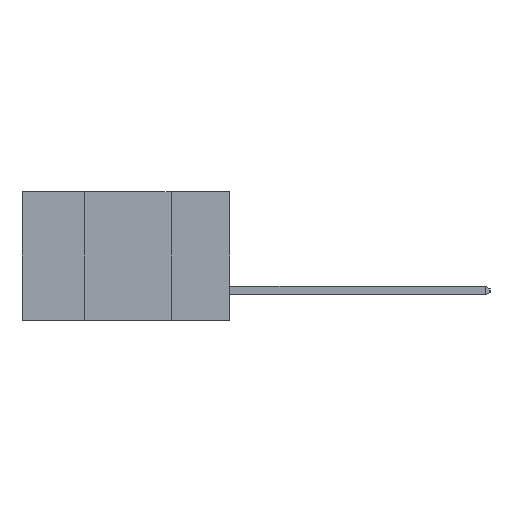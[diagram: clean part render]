
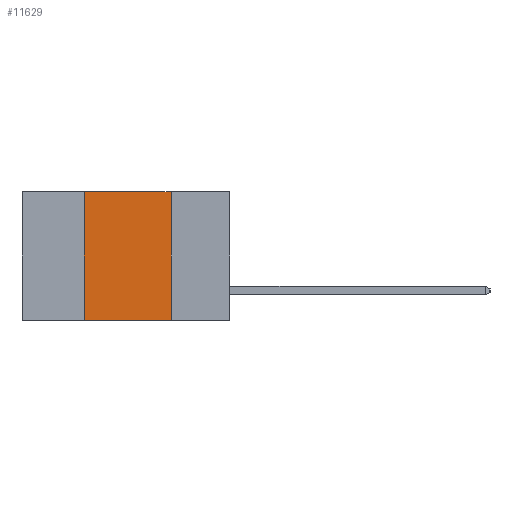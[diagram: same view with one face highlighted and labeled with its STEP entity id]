
A CAD part, left-side view. The second image highlights one B-rep face of the part: STEP entity #11629.
In plain terms, the highlighted planar face has unit normal (-1, 0, 0).
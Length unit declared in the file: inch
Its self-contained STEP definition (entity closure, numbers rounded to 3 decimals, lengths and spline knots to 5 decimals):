
#377 = CARTESIAN_POINT ( 'NONE',  ( 0., 0.42, 0. ) ) ;
#571 = DIRECTION ( 'NONE',  ( 0., -1., 0. ) ) ;
#684 = CARTESIAN_POINT ( 'NONE',  ( 0., 0.42, -0.37 ) ) ;
#943 = EDGE_LOOP ( 'NONE', ( #2612, #11514, #7344, #5136 ) ) ;
#1058 = CARTESIAN_POINT ( 'NONE',  ( 0., 0.6, -0.37 ) ) ;
#1068 = AXIS2_PLACEMENT_3D ( 'NONE', #4543, #5641, #13134 ) ;
#2128 = LINE ( 'NONE', #7784, #7578 ) ;
#2478 = EDGE_CURVE ( 'NONE', #11890, #4574, #3225, .T. ) ;
#2612 = ORIENTED_EDGE ( 'NONE', *, *, #4642, .F. ) ;
#3178 = EDGE_CURVE ( 'NONE', #11890, #9450, #10637, .T. ) ;
#3225 = LINE ( 'NONE', #1058, #5809 ) ;
#3262 = CARTESIAN_POINT ( 'NONE',  ( 0., 0.17, 0. ) ) ;
#3525 = DIRECTION ( 'NONE',  ( 0., 0., -1. ) ) ;
#4326 = CARTESIAN_POINT ( 'NONE',  ( 0., 0.42, 0. ) ) ;
#4514 = LINE ( 'NONE', #7840, #12747 ) ;
#4543 = CARTESIAN_POINT ( 'NONE',  ( 0., 0.6, 0. ) ) ;
#4574 = VERTEX_POINT ( 'NONE', #13069 ) ;
#4642 = EDGE_CURVE ( 'NONE', #6007, #4574, #4514, .T. ) ;
#4832 = DIRECTION ( 'NONE',  ( 0., 0., 1. ) ) ;
#5136 = ORIENTED_EDGE ( 'NONE', *, *, #2478, .T. ) ;
#5641 = DIRECTION ( 'NONE',  ( 1., 0., 0. ) ) ;
#5809 = VECTOR ( 'NONE', #571, 39.37008 ) ;
#6007 = VERTEX_POINT ( 'NONE', #3262 ) ;
#7032 = EDGE_CURVE ( 'NONE', #9450, #6007, #2128, .T. ) ;
#7344 = ORIENTED_EDGE ( 'NONE', *, *, #3178, .F. ) ;
#7578 = VECTOR ( 'NONE', #9942, 39.37008 ) ;
#7784 = CARTESIAN_POINT ( 'NONE',  ( 0., 0.6, 0. ) ) ;
#7840 = CARTESIAN_POINT ( 'NONE',  ( 0., 0.17, 0. ) ) ;
#9450 = VERTEX_POINT ( 'NONE', #377 ) ;
#9724 = FACE_OUTER_BOUND ( 'NONE', #943, .T. ) ;
#9942 = DIRECTION ( 'NONE',  ( 0., -1., 0. ) ) ;
#10637 = LINE ( 'NONE', #4326, #12817 ) ;
#10981 = PLANE ( 'NONE',  #1068 ) ;
#11514 = ORIENTED_EDGE ( 'NONE', *, *, #7032, .F. ) ;
#11629 = ADVANCED_FACE ( 'NONE', ( #9724 ), #10981, .F. ) ;
#11890 = VERTEX_POINT ( 'NONE', #684 ) ;
#12747 = VECTOR ( 'NONE', #3525, 39.37008 ) ;
#12817 = VECTOR ( 'NONE', #4832, 39.37008 ) ;
#13069 = CARTESIAN_POINT ( 'NONE',  ( 0., 0.17, -0.37 ) ) ;
#13134 = DIRECTION ( 'NONE',  ( 0., 0., -1. ) ) ;
